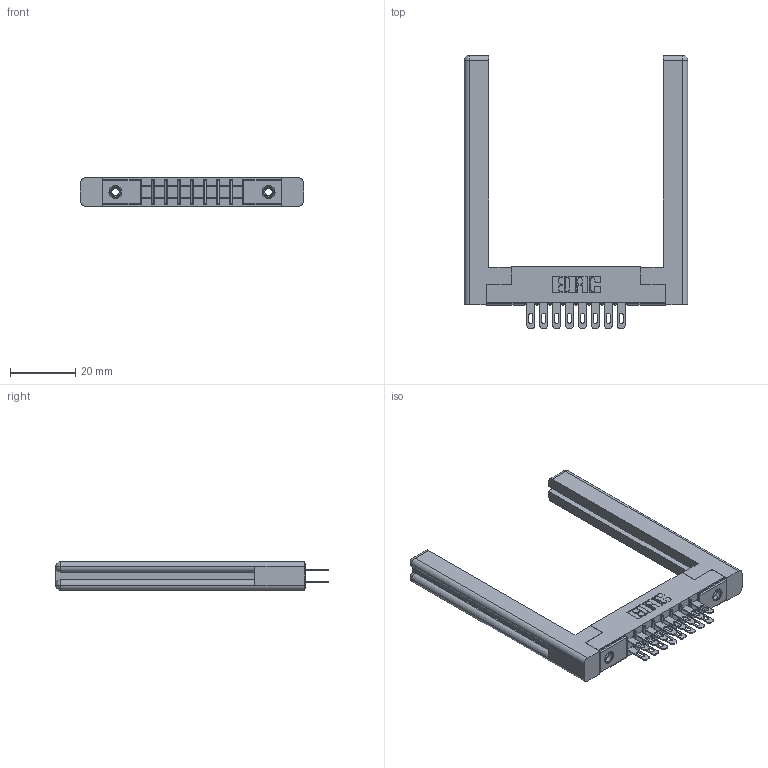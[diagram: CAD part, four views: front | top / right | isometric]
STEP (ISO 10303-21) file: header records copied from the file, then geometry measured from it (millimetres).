
FILE_DESCRIPTION (( 'STEP AP203' ), '1' );
FILE_NAME ('315-016-500-258.STEP', '2019-09-10T13:44:06', ( '' ), ( '' ), 'SwSTEP 2.0', 'SolidWorks 2016', '' );
FILE_SCHEMA (( 'CONFIG_CONTROL_DESIGN' ));
Length unit declared in the file: inch
Products named in the file (5): 315-016-500-258; 307-220-058; 345-250-001_345-250-001-102; 305-290-001_500; 305 Part_.156 Dia
Assembly tree (21 placements, depth 2):
  315-016-500-258
    305 Part_.156 Dia
    305-290-001_500  x16
    345-250-001_345-250-001-102  x2
    307-220-058  x2
Bounding box: 68.33 x 83.49 x 8.71 mm (x, y, z)
Volume: 12083.2 mm3; surface area: 12731.1 mm2
Topology: 21 solids, 21 shells, 1058 faces, 2966 edges, 1920 vertices
Faces by surface type: plane 600, cylinder 402, sphere 32, cone 12, torus 12
Entity records: 15456 total; most frequent: CARTESIAN_POINT 2573, ORIENTED_EDGE 2490, DIRECTION 2481, EDGE_CURVE 1245, VECTOR 957, LINE 957, VERTEX_POINT 800, AXIS2_PLACEMENT_3D 762
